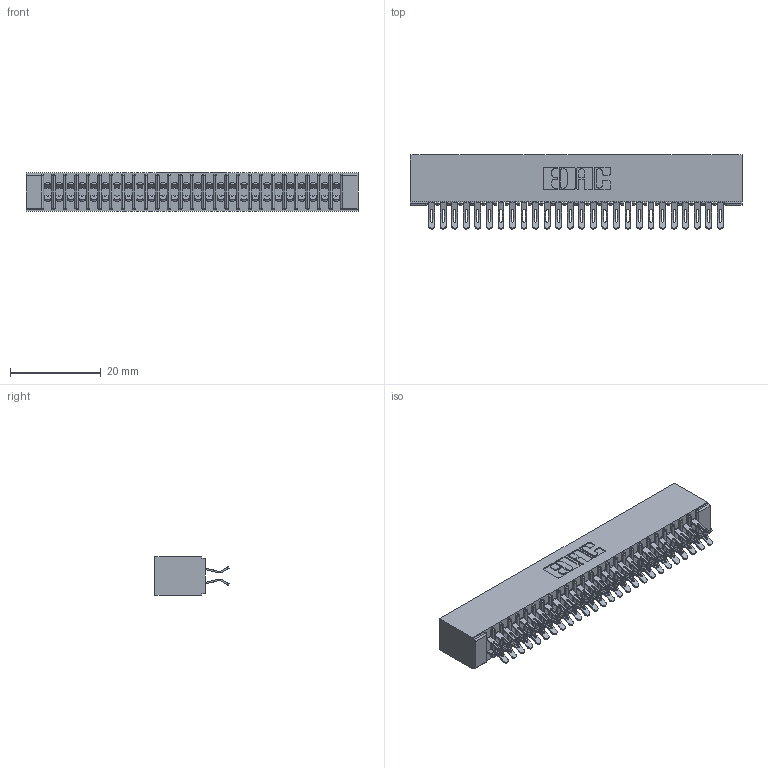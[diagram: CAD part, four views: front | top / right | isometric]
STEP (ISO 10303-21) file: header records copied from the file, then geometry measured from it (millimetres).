
FILE_DESCRIPTION (( 'STEP AP203' ), '1' );
FILE_NAME ('341-052-555-201.STEP', '2018-08-07T13:27:49', ( '' ), ( '' ), 'SwSTEP 2.0', 'SolidWorks 2016', '' );
FILE_SCHEMA (( 'CONFIG_CONTROL_DESIGN' ));
Length unit declared in the file: inch
Products named in the file (3): 341 Part_No Mounting Lugs; 341-292-001_341-292-155; 341-052-555-201
Assembly tree (53 placements, depth 2):
  341-052-555-201
    341 Part_No Mounting Lugs
    341-292-001_341-292-155  x52
Bounding box: 73.03 x 16.31 x 8.38 mm (x, y, z)
Volume: 4341.4 mm3; surface area: 10368.5 mm2
Topology: 53 solids, 53 shells, 4164 faces, 12434 edges, 8094 vertices
Faces by surface type: plane 2248, cylinder 1812, sphere 54, torus 50
Entity records: 33789 total; most frequent: CARTESIAN_POINT 5632, ORIENTED_EDGE 5584, DIRECTION 5466, EDGE_CURVE 2792, LINE 2226, VECTOR 2226, VERTEX_POINT 1770, AXIS2_PLACEMENT_3D 1620
